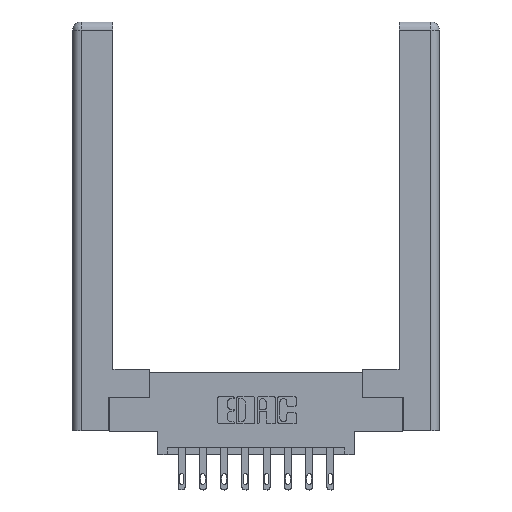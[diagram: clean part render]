
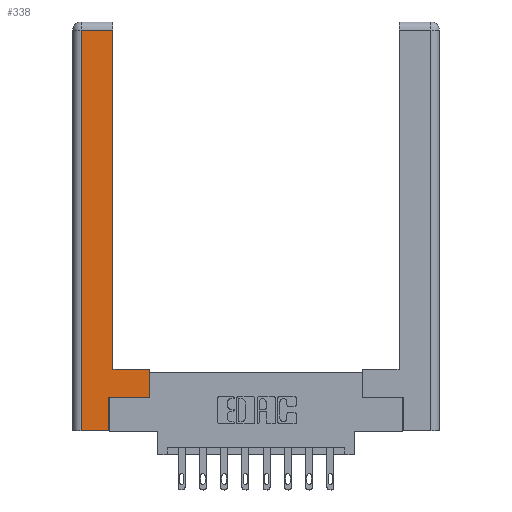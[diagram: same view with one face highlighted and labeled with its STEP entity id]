
A CAD part, top view. The second image highlights one B-rep face of the part: STEP entity #338.
In plain terms, the highlighted planar face has unit normal (0, 0, 1).
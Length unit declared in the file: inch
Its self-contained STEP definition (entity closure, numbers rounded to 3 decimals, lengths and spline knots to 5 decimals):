
#87 = ORIENTED_EDGE ( 'NONE', *, *, #6169, .T. ) ;
#88 = CARTESIAN_POINT ( 'NONE',  ( 0.565, 0.245, 0. ) ) ;
#187 = DIRECTION ( 'NONE',  ( 1., 0., 0. ) ) ;
#338 = ADVANCED_FACE ( 'NONE', ( #11146 ), #12912, .F. ) ;
#544 = DIRECTION ( 'NONE',  ( 1., 0., 0. ) ) ;
#970 = LINE ( 'NONE', #11058, #10782 ) ;
#1239 = LINE ( 'NONE', #8887, #3328 ) ;
#1550 = EDGE_CURVE ( 'NONE', #4722, #4629, #6829, .T. ) ;
#1642 = DIRECTION ( 'NONE',  ( 0., 0., -1. ) ) ;
#2165 = EDGE_CURVE ( 'NONE', #8232, #4722, #8392, .T. ) ;
#2213 = CARTESIAN_POINT ( 'NONE',  ( 0.0615, 0., 0. ) ) ;
#2227 = ORIENTED_EDGE ( 'NONE', *, *, #5873, .T. ) ;
#3214 = DIRECTION ( 'NONE',  ( 0., 1., 0. ) ) ;
#3328 = VECTOR ( 'NONE', #8930, 39.37008 ) ;
#3632 = CARTESIAN_POINT ( 'NONE',  ( 0.265, 0.245, 0. ) ) ;
#3692 = VECTOR ( 'NONE', #544, 39.37008 ) ;
#4071 = CARTESIAN_POINT ( 'NONE',  ( 0.0615, 2.94, 0. ) ) ;
#4127 = DIRECTION ( 'NONE',  ( 0., 1., 0. ) ) ;
#4130 = ORIENTED_EDGE ( 'NONE', *, *, #9857, .T. ) ;
#4147 = CARTESIAN_POINT ( 'NONE',  ( 0.0615, 2.94, 0. ) ) ;
#4207 = CARTESIAN_POINT ( 'NONE',  ( 0.295, 0.45, 0. ) ) ;
#4349 = CARTESIAN_POINT ( 'NONE',  ( 0.565, 0.45, 0. ) ) ;
#4364 = LINE ( 'NONE', #4147, #6138 ) ;
#4629 = VERTEX_POINT ( 'NONE', #4207 ) ;
#4722 = VERTEX_POINT ( 'NONE', #4349 ) ;
#5038 = CARTESIAN_POINT ( 'NONE',  ( 0.295, 0.45, 0. ) ) ;
#5323 = LINE ( 'NONE', #8686, #3692 ) ;
#5794 = DIRECTION ( 'NONE',  ( -1., 0., 0. ) ) ;
#5873 = EDGE_CURVE ( 'NONE', #10933, #10485, #1239, .T. ) ;
#6138 = VECTOR ( 'NONE', #11181, 39.37008 ) ;
#6169 = EDGE_CURVE ( 'NONE', #10485, #8980, #9436, .T. ) ;
#6504 = CARTESIAN_POINT ( 'NONE',  ( 0.265, 0., 0. ) ) ;
#6829 = LINE ( 'NONE', #5038, #8555 ) ;
#7021 = VERTEX_POINT ( 'NONE', #3632 ) ;
#7190 = CARTESIAN_POINT ( 'NONE',  ( 0.295, 2.94, 0. ) ) ;
#7373 = CARTESIAN_POINT ( 'NONE',  ( 0.565, 0.45, 0. ) ) ;
#7474 = AXIS2_PLACEMENT_3D ( 'NONE', #7822, #1642, #5794 ) ;
#7740 = ORIENTED_EDGE ( 'NONE', *, *, #11040, .T. ) ;
#7822 = CARTESIAN_POINT ( 'NONE',  ( 0., 0., 0. ) ) ;
#8039 = DIRECTION ( 'NONE',  ( 0., 1., 0. ) ) ;
#8232 = VERTEX_POINT ( 'NONE', #88 ) ;
#8341 = ORIENTED_EDGE ( 'NONE', *, *, #9256, .T. ) ;
#8392 = LINE ( 'NONE', #7373, #11105 ) ;
#8555 = VECTOR ( 'NONE', #10286, 39.37008 ) ;
#8686 = CARTESIAN_POINT ( 'NONE',  ( 0.565, 0.245, 0. ) ) ;
#8845 = ORIENTED_EDGE ( 'NONE', *, *, #1550, .T. ) ;
#8887 = CARTESIAN_POINT ( 'NONE',  ( 0.0615, 0., 0. ) ) ;
#8930 = DIRECTION ( 'NONE',  ( 0., -1., 0. ) ) ;
#8980 = VERTEX_POINT ( 'NONE', #6504 ) ;
#9256 = EDGE_CURVE ( 'NONE', #4629, #10207, #970, .T. ) ;
#9308 = ORIENTED_EDGE ( 'NONE', *, *, #2165, .T. ) ;
#9436 = LINE ( 'NONE', #12445, #10563 ) ;
#9857 = EDGE_CURVE ( 'NONE', #8980, #7021, #10059, .T. ) ;
#10059 = LINE ( 'NONE', #10584, #12455 ) ;
#10207 = VERTEX_POINT ( 'NONE', #7190 ) ;
#10286 = DIRECTION ( 'NONE',  ( -1., 0., 0. ) ) ;
#10485 = VERTEX_POINT ( 'NONE', #2213 ) ;
#10553 = ORIENTED_EDGE ( 'NONE', *, *, #11395, .T. ) ;
#10563 = VECTOR ( 'NONE', #187, 39.37008 ) ;
#10584 = CARTESIAN_POINT ( 'NONE',  ( 0.265, 0.245, 0. ) ) ;
#10782 = VECTOR ( 'NONE', #8039, 39.37008 ) ;
#10933 = VERTEX_POINT ( 'NONE', #4071 ) ;
#11040 = EDGE_CURVE ( 'NONE', #10207, #10933, #4364, .T. ) ;
#11058 = CARTESIAN_POINT ( 'NONE',  ( 0.295, 3., 0. ) ) ;
#11105 = VECTOR ( 'NONE', #4127, 39.37008 ) ;
#11146 = FACE_OUTER_BOUND ( 'NONE', #13265, .T. ) ;
#11181 = DIRECTION ( 'NONE',  ( -1., 0., 0. ) ) ;
#11395 = EDGE_CURVE ( 'NONE', #7021, #8232, #5323, .T. ) ;
#12445 = CARTESIAN_POINT ( 'NONE',  ( 0.265, 0., 0. ) ) ;
#12455 = VECTOR ( 'NONE', #3214, 39.37008 ) ;
#12912 = PLANE ( 'NONE',  #7474 ) ;
#13265 = EDGE_LOOP ( 'NONE', ( #8341, #7740, #2227, #87, #4130, #10553, #9308, #8845 ) ) ;
